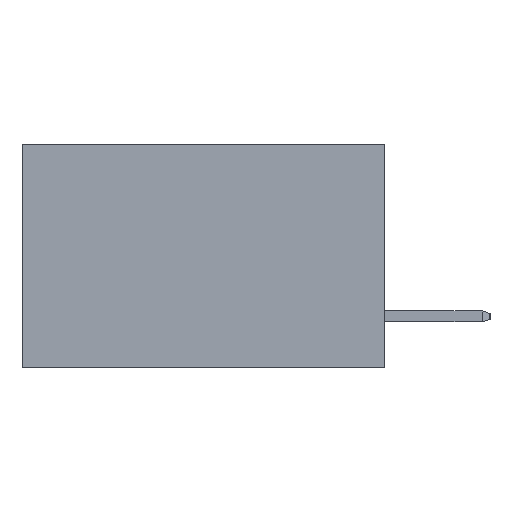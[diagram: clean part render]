
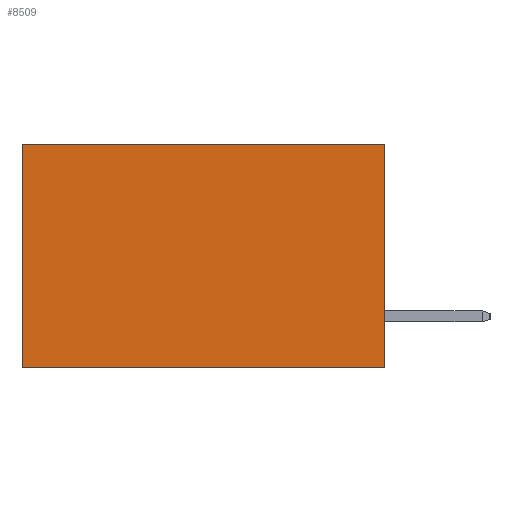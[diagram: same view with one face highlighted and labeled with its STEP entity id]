
A CAD part, left-side view. The second image highlights one B-rep face of the part: STEP entity #8509.
In plain terms, the highlighted planar face has unit normal (-1, 0, 0).
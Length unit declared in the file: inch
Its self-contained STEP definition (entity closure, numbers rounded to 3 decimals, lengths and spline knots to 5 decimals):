
#9 = DIRECTION ( 'NONE',  ( 1., 0., 0. ) ) ;
#130 = VERTEX_POINT ( 'NONE', #3520 ) ;
#212 = CARTESIAN_POINT ( 'NONE',  ( 0.298, 0., 0. ) ) ;
#592 = EDGE_CURVE ( 'NONE', #10608, #10995, #10639, .T. ) ;
#1870 = CARTESIAN_POINT ( 'NONE',  ( 0.298, 0., 0. ) ) ;
#1877 = DIRECTION ( 'NONE',  ( 0., 1., 0. ) ) ;
#2344 = PLANE ( 'NONE',  #9754 ) ;
#2461 = CARTESIAN_POINT ( 'NONE',  ( 0.298, 0., -0.37 ) ) ;
#2694 = LINE ( 'NONE', #1870, #5606 ) ;
#3227 = CARTESIAN_POINT ( 'NONE',  ( 0.298, 0.6, -0.37 ) ) ;
#3349 = VECTOR ( 'NONE', #3981, 39.37008 ) ;
#3520 = CARTESIAN_POINT ( 'NONE',  ( 0.298, 0., 0. ) ) ;
#3981 = DIRECTION ( 'NONE',  ( 0., 0., -1. ) ) ;
#5606 = VECTOR ( 'NONE', #1877, 39.37008 ) ;
#5855 = ORIENTED_EDGE ( 'NONE', *, *, #592, .F. ) ;
#6657 = LINE ( 'NONE', #8938, #3349 ) ;
#6706 = EDGE_CURVE ( 'NONE', #130, #14714, #2694, .T. ) ;
#6863 = DIRECTION ( 'NONE',  ( 0., 0., -1. ) ) ;
#7604 = ORIENTED_EDGE ( 'NONE', *, *, #10746, .F. ) ;
#8032 = CARTESIAN_POINT ( 'NONE',  ( 0.298, 0.6, 0. ) ) ;
#8052 = DIRECTION ( 'NONE',  ( 0., 0., -1. ) ) ;
#8509 = ADVANCED_FACE ( 'NONE', ( #15488 ), #2344, .F. ) ;
#8874 = EDGE_CURVE ( 'NONE', #14714, #10995, #11579, .T. ) ;
#8938 = CARTESIAN_POINT ( 'NONE',  ( 0.298, 0., 0. ) ) ;
#9754 = AXIS2_PLACEMENT_3D ( 'NONE', #212, #9, #6863 ) ;
#10381 = VECTOR ( 'NONE', #8052, 39.37008 ) ;
#10608 = VERTEX_POINT ( 'NONE', #2461 ) ;
#10639 = LINE ( 'NONE', #14841, #13606 ) ;
#10746 = EDGE_CURVE ( 'NONE', #130, #10608, #6657, .T. ) ;
#10995 = VERTEX_POINT ( 'NONE', #3227 ) ;
#11579 = LINE ( 'NONE', #8032, #10381 ) ;
#12219 = ORIENTED_EDGE ( 'NONE', *, *, #8874, .T. ) ;
#13341 = CARTESIAN_POINT ( 'NONE',  ( 0.298, 0.6, 0. ) ) ;
#13606 = VECTOR ( 'NONE', #14909, 39.37008 ) ;
#14714 = VERTEX_POINT ( 'NONE', #13341 ) ;
#14841 = CARTESIAN_POINT ( 'NONE',  ( 0.298, 0., -0.37 ) ) ;
#14909 = DIRECTION ( 'NONE',  ( 0., 1., 0. ) ) ;
#15289 = ORIENTED_EDGE ( 'NONE', *, *, #6706, .T. ) ;
#15296 = EDGE_LOOP ( 'NONE', ( #12219, #5855, #7604, #15289 ) ) ;
#15488 = FACE_OUTER_BOUND ( 'NONE', #15296, .T. ) ;
